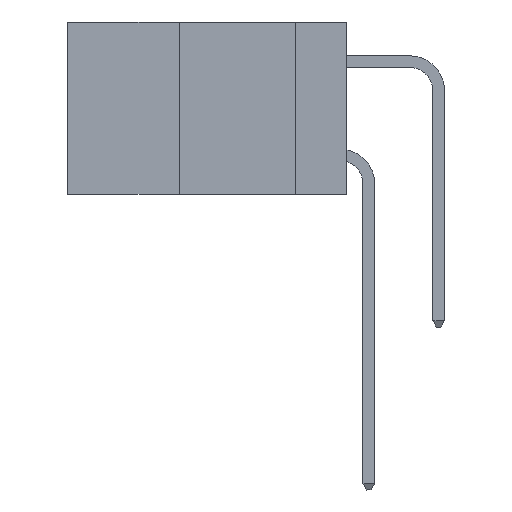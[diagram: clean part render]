
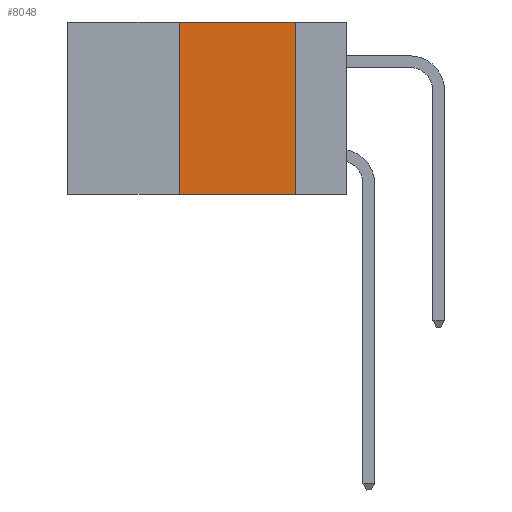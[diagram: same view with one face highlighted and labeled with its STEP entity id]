
A CAD part, left-side view. The second image highlights one B-rep face of the part: STEP entity #8048.
In plain terms, the highlighted planar face has unit normal (-1, 0, 0).
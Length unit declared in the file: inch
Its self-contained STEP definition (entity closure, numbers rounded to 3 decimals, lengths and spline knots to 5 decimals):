
#228 = VECTOR ( 'NONE', #10951, 39.37008 ) ;
#231 = EDGE_LOOP ( 'NONE', ( #349, #3870, #1429, #11266 ) ) ;
#296 = VECTOR ( 'NONE', #6393, 39.37008 ) ;
#349 = ORIENTED_EDGE ( 'NONE', *, *, #4023, .F. ) ;
#434 = DIRECTION ( 'NONE',  ( 0., 0., -1. ) ) ;
#514 = CARTESIAN_POINT ( 'NONE',  ( 0., 0.11, 0. ) ) ;
#839 = DIRECTION ( 'NONE',  ( 0., 0., -1. ) ) ;
#1005 = VERTEX_POINT ( 'NONE', #6787 ) ;
#1429 = ORIENTED_EDGE ( 'NONE', *, *, #10145, .F. ) ;
#1673 = CARTESIAN_POINT ( 'NONE',  ( 0., 0.6, 0. ) ) ;
#2941 = LINE ( 'NONE', #6419, #228 ) ;
#3160 = VERTEX_POINT ( 'NONE', #7192 ) ;
#3742 = CARTESIAN_POINT ( 'NONE',  ( 0., 0.36, -0.37 ) ) ;
#3870 = ORIENTED_EDGE ( 'NONE', *, *, #8976, .F. ) ;
#4023 = EDGE_CURVE ( 'NONE', #3160, #7202, #6588, .T. ) ;
#5551 = LINE ( 'NONE', #1673, #296 ) ;
#5814 = EDGE_CURVE ( 'NONE', #9830, #7202, #2941, .T. ) ;
#6320 = VECTOR ( 'NONE', #434, 39.37008 ) ;
#6393 = DIRECTION ( 'NONE',  ( 0., -1., 0. ) ) ;
#6419 = CARTESIAN_POINT ( 'NONE',  ( 0., 0.6, -0.37 ) ) ;
#6541 = AXIS2_PLACEMENT_3D ( 'NONE', #10193, #6573, #839 ) ;
#6573 = DIRECTION ( 'NONE',  ( 1., 0., 0. ) ) ;
#6588 = LINE ( 'NONE', #514, #6320 ) ;
#6787 = CARTESIAN_POINT ( 'NONE',  ( 0., 0.36, 0. ) ) ;
#7192 = CARTESIAN_POINT ( 'NONE',  ( 0., 0.11, 0. ) ) ;
#7202 = VERTEX_POINT ( 'NONE', #10850 ) ;
#8048 = ADVANCED_FACE ( 'NONE', ( #11766 ), #11888, .F. ) ;
#8534 = VECTOR ( 'NONE', #9548, 39.37008 ) ;
#8976 = EDGE_CURVE ( 'NONE', #1005, #3160, #5551, .T. ) ;
#9548 = DIRECTION ( 'NONE',  ( 0., 0., 1. ) ) ;
#9830 = VERTEX_POINT ( 'NONE', #3742 ) ;
#10145 = EDGE_CURVE ( 'NONE', #9830, #1005, #10946, .T. ) ;
#10193 = CARTESIAN_POINT ( 'NONE',  ( 0., 0.6, 0. ) ) ;
#10850 = CARTESIAN_POINT ( 'NONE',  ( 0., 0.11, -0.37 ) ) ;
#10946 = LINE ( 'NONE', #11347, #8534 ) ;
#10951 = DIRECTION ( 'NONE',  ( 0., -1., 0. ) ) ;
#11266 = ORIENTED_EDGE ( 'NONE', *, *, #5814, .T. ) ;
#11347 = CARTESIAN_POINT ( 'NONE',  ( 0., 0.36, 0. ) ) ;
#11766 = FACE_OUTER_BOUND ( 'NONE', #231, .T. ) ;
#11888 = PLANE ( 'NONE',  #6541 ) ;
